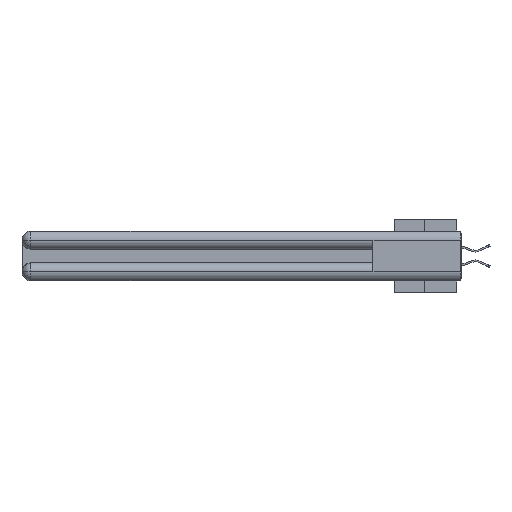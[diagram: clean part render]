
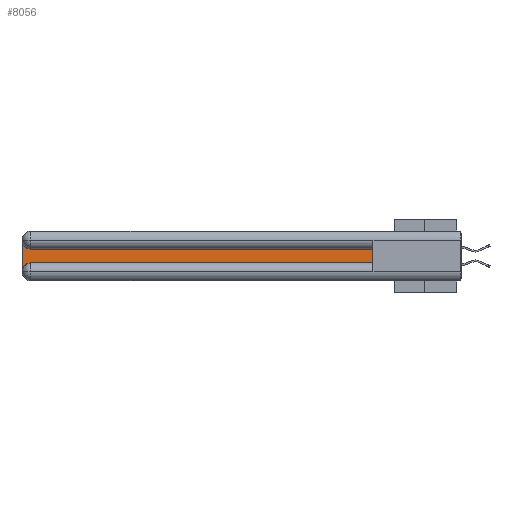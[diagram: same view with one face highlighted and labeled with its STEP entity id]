
A CAD part, left-side view. The second image highlights one B-rep face of the part: STEP entity #8056.
In plain terms, the highlighted planar face has unit normal (-1, 0, 0).
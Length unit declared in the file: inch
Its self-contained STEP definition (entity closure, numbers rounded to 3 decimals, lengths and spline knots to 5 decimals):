
#1351 = DIRECTION ( 'NONE',  ( 1., 0., 0. ) ) ;
#1443 = VERTEX_POINT ( 'NONE', #22946 ) ;
#2561 = FACE_OUTER_BOUND ( 'NONE', #30807, .T. ) ;
#3410 = ORIENTED_EDGE ( 'NONE', *, *, #17549, .T. ) ;
#3751 = VECTOR ( 'NONE', #16853, 39.37008 ) ;
#4819 = CARTESIAN_POINT ( 'NONE',  ( 0.075, 0.6, -0.1225 ) ) ;
#5425 = LINE ( 'NONE', #29380, #32342 ) ;
#5450 = ORIENTED_EDGE ( 'NONE', *, *, #34965, .T. ) ;
#5767 = CARTESIAN_POINT ( 'NONE',  ( 0.075, 3., -0.1225 ) ) ;
#8056 = ADVANCED_FACE ( 'NONE', ( #2561 ), #9128, .F. ) ;
#9128 = PLANE ( 'NONE',  #18168 ) ;
#9227 = DIRECTION ( 'NONE',  ( 0., 0., 1. ) ) ;
#11291 = ORIENTED_EDGE ( 'NONE', *, *, #22900, .T. ) ;
#11796 = CARTESIAN_POINT ( 'NONE',  ( 0.075, 2.94, -0.2775 ) ) ;
#11833 = DIRECTION ( 'NONE',  ( 0., 0., -1. ) ) ;
#12005 = DIRECTION ( 'NONE',  ( 0., 1., 0. ) ) ;
#12392 = DIRECTION ( 'NONE',  ( 1., 0., 0. ) ) ;
#13881 = CARTESIAN_POINT ( 'NONE',  ( 0.075, 0.6, -0.2175 ) ) ;
#14730 = CARTESIAN_POINT ( 'NONE',  ( 0.075, 0.6, -0.2175 ) ) ;
#15686 = CARTESIAN_POINT ( 'NONE',  ( 0.075, 2.94, -0.1225 ) ) ;
#15974 = DIRECTION ( 'NONE',  ( 0., 0., -1. ) ) ;
#16151 = LINE ( 'NONE', #16298, #19468 ) ;
#16298 = CARTESIAN_POINT ( 'NONE',  ( 0.075, 0.6, -0.2175 ) ) ;
#16769 = EDGE_CURVE ( 'NONE', #41158, #40280, #39877, .T. ) ;
#16853 = DIRECTION ( 'NONE',  ( 0., -1., 0. ) ) ;
#17549 = EDGE_CURVE ( 'NONE', #23753, #1443, #20088, .T. ) ;
#17988 = CARTESIAN_POINT ( 'NONE',  ( 0.075, 3., -0.2775 ) ) ;
#18168 = AXIS2_PLACEMENT_3D ( 'NONE', #5767, #19438, #40731 ) ;
#18224 = ORIENTED_EDGE ( 'NONE', *, *, #38214, .T. ) ;
#18543 = CARTESIAN_POINT ( 'NONE',  ( 0.075, 2.94, -0.0625 ) ) ;
#19283 = VERTEX_POINT ( 'NONE', #14730 ) ;
#19438 = DIRECTION ( 'NONE',  ( 1., 0., 0. ) ) ;
#19468 = VECTOR ( 'NONE', #9227, 39.37008 ) ;
#20088 = CIRCLE ( 'NONE', #25231, 0.06 ) ;
#22900 = EDGE_CURVE ( 'NONE', #1443, #19283, #38853, .T. ) ;
#22946 = CARTESIAN_POINT ( 'NONE',  ( 0.075, 2.94, -0.2175 ) ) ;
#23753 = VERTEX_POINT ( 'NONE', #17988 ) ;
#25231 = AXIS2_PLACEMENT_3D ( 'NONE', #11796, #12392, #15974 ) ;
#27447 = ORIENTED_EDGE ( 'NONE', *, *, #45254, .T. ) ;
#28343 = LINE ( 'NONE', #4819, #34953 ) ;
#29380 = CARTESIAN_POINT ( 'NONE',  ( 0.075, 3., -0.2175 ) ) ;
#30080 = ORIENTED_EDGE ( 'NONE', *, *, #16769, .T. ) ;
#30807 = EDGE_LOOP ( 'NONE', ( #27447, #30080, #18224, #3410, #11291, #5450 ) ) ;
#32342 = VECTOR ( 'NONE', #11833, 39.37008 ) ;
#34902 = CARTESIAN_POINT ( 'NONE',  ( 0.075, 3., -0.0625 ) ) ;
#34953 = VECTOR ( 'NONE', #12005, 39.37008 ) ;
#34965 = EDGE_CURVE ( 'NONE', #19283, #40970, #16151, .T. ) ;
#35811 = AXIS2_PLACEMENT_3D ( 'NONE', #18543, #1351, #44296 ) ;
#37511 = CARTESIAN_POINT ( 'NONE',  ( 0.075, 0.6, -0.1225 ) ) ;
#38214 = EDGE_CURVE ( 'NONE', #40280, #23753, #5425, .T. ) ;
#38853 = LINE ( 'NONE', #13881, #3751 ) ;
#39877 = CIRCLE ( 'NONE', #35811, 0.06 ) ;
#40280 = VERTEX_POINT ( 'NONE', #34902 ) ;
#40731 = DIRECTION ( 'NONE',  ( 0., 0., -1. ) ) ;
#40970 = VERTEX_POINT ( 'NONE', #37511 ) ;
#41158 = VERTEX_POINT ( 'NONE', #15686 ) ;
#44296 = DIRECTION ( 'NONE',  ( 0., 0., -1. ) ) ;
#45254 = EDGE_CURVE ( 'NONE', #40970, #41158, #28343, .T. ) ;
